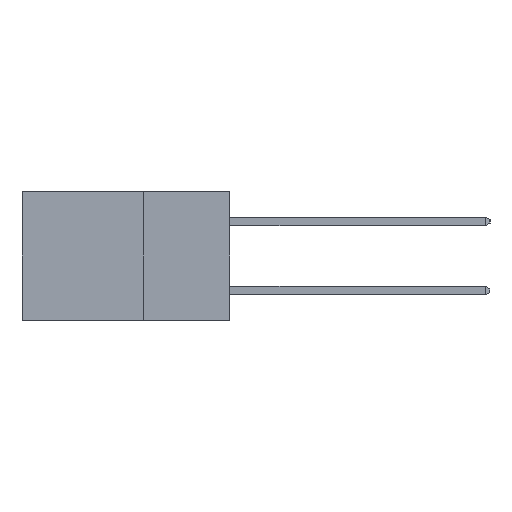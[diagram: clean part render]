
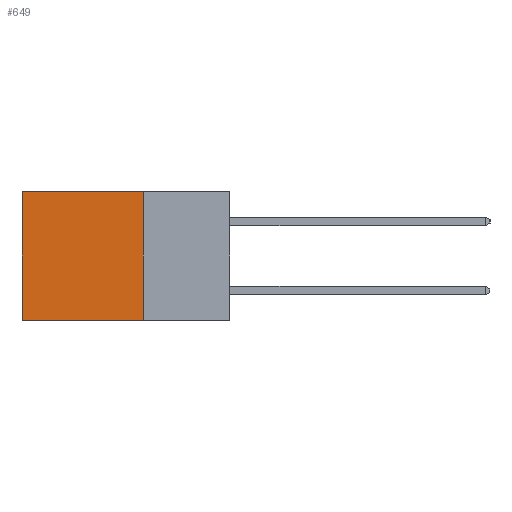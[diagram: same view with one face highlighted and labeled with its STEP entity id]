
A CAD part, left-side view. The second image highlights one B-rep face of the part: STEP entity #649.
In plain terms, the highlighted planar face has unit normal (-1, 0, 0).
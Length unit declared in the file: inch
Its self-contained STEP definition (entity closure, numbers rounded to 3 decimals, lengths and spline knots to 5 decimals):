
#253 = CARTESIAN_POINT ( 'NONE',  ( 0.298, 0.6, -0.37 ) ) ;
#417 = EDGE_LOOP ( 'NONE', ( #2686, #15547, #2093, #14416 ) ) ;
#649 = ADVANCED_FACE ( 'NONE', ( #12931 ), #12301, .F. ) ;
#2093 = ORIENTED_EDGE ( 'NONE', *, *, #6609, .F. ) ;
#2469 = EDGE_CURVE ( 'NONE', #15003, #11111, #5649, .T. ) ;
#2686 = ORIENTED_EDGE ( 'NONE', *, *, #15165, .T. ) ;
#3715 = EDGE_CURVE ( 'NONE', #16126, #11261, #16488, .T. ) ;
#4159 = CARTESIAN_POINT ( 'NONE',  ( 0.298, 0.25, 0. ) ) ;
#4484 = LINE ( 'NONE', #4159, #7138 ) ;
#5134 = CARTESIAN_POINT ( 'NONE',  ( 0.298, 0.6, 0. ) ) ;
#5563 = DIRECTION ( 'NONE',  ( 0., 0., -1. ) ) ;
#5649 = LINE ( 'NONE', #5660, #12277 ) ;
#5660 = CARTESIAN_POINT ( 'NONE',  ( 0.298, 0.25, 0. ) ) ;
#6609 = EDGE_CURVE ( 'NONE', #15003, #16126, #4484, .T. ) ;
#7138 = VECTOR ( 'NONE', #5563, 39.37008 ) ;
#7419 = CARTESIAN_POINT ( 'NONE',  ( 0.298, 0.25, -0.37 ) ) ;
#7807 = DIRECTION ( 'NONE',  ( 0., 1., 0. ) ) ;
#7908 = DIRECTION ( 'NONE',  ( 0., 0., -1. ) ) ;
#8930 = CARTESIAN_POINT ( 'NONE',  ( 0.298, 0.25, 0. ) ) ;
#9564 = LINE ( 'NONE', #5134, #16096 ) ;
#11111 = VERTEX_POINT ( 'NONE', #16230 ) ;
#11261 = VERTEX_POINT ( 'NONE', #253 ) ;
#11982 = DIRECTION ( 'NONE',  ( 0., 0., -1. ) ) ;
#12277 = VECTOR ( 'NONE', #7807, 39.37008 ) ;
#12301 = PLANE ( 'NONE',  #13450 ) ;
#12317 = DIRECTION ( 'NONE',  ( 0., 1., 0. ) ) ;
#12931 = FACE_OUTER_BOUND ( 'NONE', #417, .T. ) ;
#13029 = VECTOR ( 'NONE', #12317, 39.37008 ) ;
#13450 = AXIS2_PLACEMENT_3D ( 'NONE', #15239, #14376, #11982 ) ;
#13695 = CARTESIAN_POINT ( 'NONE',  ( 0.298, 0.25, -0.37 ) ) ;
#14376 = DIRECTION ( 'NONE',  ( 1., 0., 0. ) ) ;
#14416 = ORIENTED_EDGE ( 'NONE', *, *, #2469, .T. ) ;
#15003 = VERTEX_POINT ( 'NONE', #8930 ) ;
#15165 = EDGE_CURVE ( 'NONE', #11111, #11261, #9564, .T. ) ;
#15239 = CARTESIAN_POINT ( 'NONE',  ( 0.298, 0.25, 0. ) ) ;
#15547 = ORIENTED_EDGE ( 'NONE', *, *, #3715, .F. ) ;
#16096 = VECTOR ( 'NONE', #7908, 39.37008 ) ;
#16126 = VERTEX_POINT ( 'NONE', #13695 ) ;
#16230 = CARTESIAN_POINT ( 'NONE',  ( 0.298, 0.6, 0. ) ) ;
#16488 = LINE ( 'NONE', #7419, #13029 ) ;
